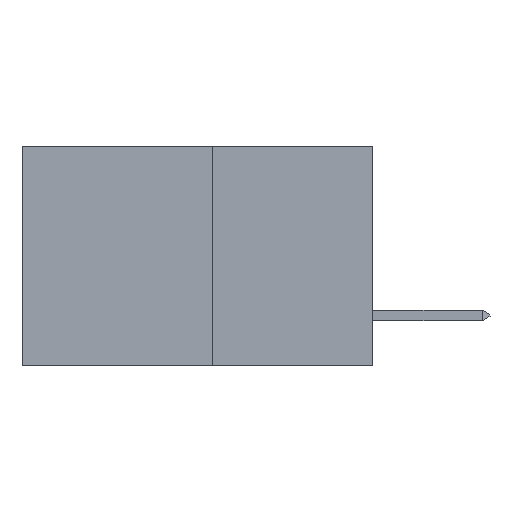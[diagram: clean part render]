
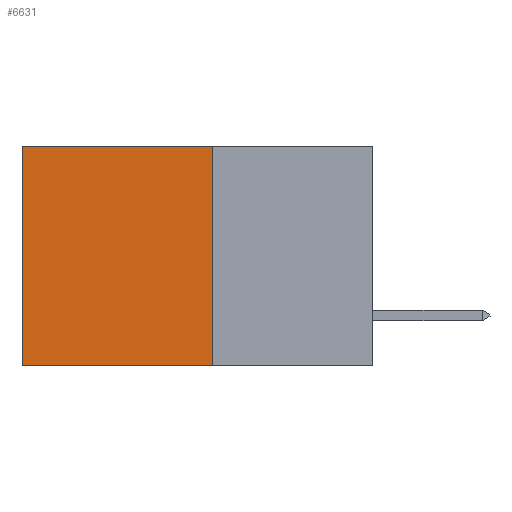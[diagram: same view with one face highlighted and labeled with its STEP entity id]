
A CAD part, left-side view. The second image highlights one B-rep face of the part: STEP entity #6631.
In plain terms, the highlighted planar face has unit normal (-1, 0, 0).
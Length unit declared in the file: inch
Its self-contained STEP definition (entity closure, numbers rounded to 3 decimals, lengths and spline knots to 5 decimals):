
#329 = CARTESIAN_POINT ( 'NONE',  ( 0.277, 0.27, -0.37 ) ) ;
#699 = ORIENTED_EDGE ( 'NONE', *, *, #857, .T. ) ;
#748 = VECTOR ( 'NONE', #3483, 39.37008 ) ;
#857 = EDGE_CURVE ( 'NONE', #1542, #7004, #2044, .T. ) ;
#1021 = PLANE ( 'NONE',  #7899 ) ;
#1056 = DIRECTION ( 'NONE',  ( 0., 0., -1. ) ) ;
#1542 = VERTEX_POINT ( 'NONE', #5020 ) ;
#2044 = LINE ( 'NONE', #8465, #5371 ) ;
#2272 = VECTOR ( 'NONE', #5849, 39.37008 ) ;
#2307 = EDGE_LOOP ( 'NONE', ( #699, #8502, #4522, #2393 ) ) ;
#2393 = ORIENTED_EDGE ( 'NONE', *, *, #5032, .T. ) ;
#2782 = DIRECTION ( 'NONE',  ( 0., 0., -1. ) ) ;
#2886 = CARTESIAN_POINT ( 'NONE',  ( 0.277, 0.59, -0.37 ) ) ;
#3145 = CARTESIAN_POINT ( 'NONE',  ( 0.277, 0.27, -0.37 ) ) ;
#3199 = EDGE_CURVE ( 'NONE', #6565, #7004, #4832, .T. ) ;
#3483 = DIRECTION ( 'NONE',  ( 0., 1., 0. ) ) ;
#4522 = ORIENTED_EDGE ( 'NONE', *, *, #6292, .F. ) ;
#4774 = LINE ( 'NONE', #5557, #748 ) ;
#4794 = CARTESIAN_POINT ( 'NONE',  ( 0.277, 0.27, -0.37 ) ) ;
#4832 = LINE ( 'NONE', #4794, #2272 ) ;
#4958 = VECTOR ( 'NONE', #2782, 39.37008 ) ;
#5020 = CARTESIAN_POINT ( 'NONE',  ( 0.277, 0.59, 0. ) ) ;
#5032 = EDGE_CURVE ( 'NONE', #5412, #1542, #4774, .T. ) ;
#5313 = DIRECTION ( 'NONE',  ( 1., 0., 0. ) ) ;
#5371 = VECTOR ( 'NONE', #8874, 39.37008 ) ;
#5373 = FACE_OUTER_BOUND ( 'NONE', #2307, .T. ) ;
#5412 = VERTEX_POINT ( 'NONE', #6036 ) ;
#5557 = CARTESIAN_POINT ( 'NONE',  ( 0.277, 0.27, 0. ) ) ;
#5849 = DIRECTION ( 'NONE',  ( 0., 1., 0. ) ) ;
#6036 = CARTESIAN_POINT ( 'NONE',  ( 0.277, 0.27, 0. ) ) ;
#6292 = EDGE_CURVE ( 'NONE', #5412, #6565, #6793, .T. ) ;
#6565 = VERTEX_POINT ( 'NONE', #3145 ) ;
#6631 = ADVANCED_FACE ( 'NONE', ( #5373 ), #1021, .F. ) ;
#6793 = LINE ( 'NONE', #9044, #4958 ) ;
#7004 = VERTEX_POINT ( 'NONE', #2886 ) ;
#7899 = AXIS2_PLACEMENT_3D ( 'NONE', #329, #5313, #1056 ) ;
#8465 = CARTESIAN_POINT ( 'NONE',  ( 0.277, 0.59, -0.37 ) ) ;
#8502 = ORIENTED_EDGE ( 'NONE', *, *, #3199, .F. ) ;
#8874 = DIRECTION ( 'NONE',  ( 0., 0., -1. ) ) ;
#9044 = CARTESIAN_POINT ( 'NONE',  ( 0.277, 0.27, -0.37 ) ) ;
